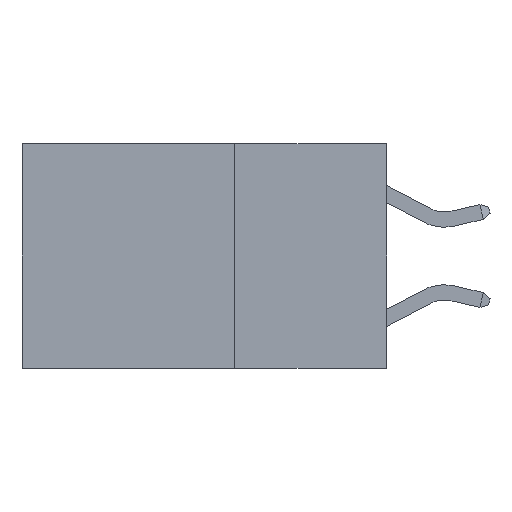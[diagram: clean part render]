
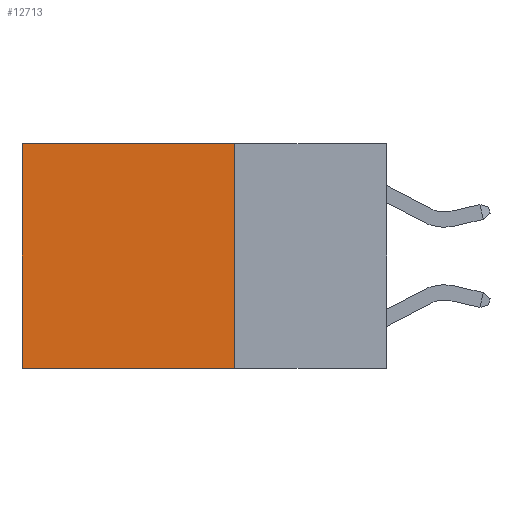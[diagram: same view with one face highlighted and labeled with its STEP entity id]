
A CAD part, left-side view. The second image highlights one B-rep face of the part: STEP entity #12713.
In plain terms, the highlighted planar face has unit normal (-1, 0, 0).
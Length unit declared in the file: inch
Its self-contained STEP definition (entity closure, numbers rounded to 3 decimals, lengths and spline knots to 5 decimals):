
#33 = EDGE_CURVE ( 'NONE', #10007, #8525, #7370, .T. ) ;
#2147 = VECTOR ( 'NONE', #4377, 39.37008 ) ;
#2740 = AXIS2_PLACEMENT_3D ( 'NONE', #23702, #5117, #19915 ) ;
#2826 = LINE ( 'NONE', #7041, #7732 ) ;
#2960 = DIRECTION ( 'NONE',  ( 0., 0., -1. ) ) ;
#3546 = CARTESIAN_POINT ( 'NONE',  ( 0.2625, 0.25, 0. ) ) ;
#3623 = EDGE_CURVE ( 'NONE', #10125, #24900, #12523, .T. ) ;
#3846 = CARTESIAN_POINT ( 'NONE',  ( 0.2625, 0.25, 0. ) ) ;
#4236 = ORIENTED_EDGE ( 'NONE', *, *, #3623, .F. ) ;
#4377 = DIRECTION ( 'NONE',  ( 0., 1., 0. ) ) ;
#5117 = DIRECTION ( 'NONE',  ( 1., 0., 0. ) ) ;
#5480 = DIRECTION ( 'NONE',  ( 0., 0., -1. ) ) ;
#7041 = CARTESIAN_POINT ( 'NONE',  ( 0.2625, 0.6, 0. ) ) ;
#7370 = LINE ( 'NONE', #3546, #26681 ) ;
#7568 = EDGE_CURVE ( 'NONE', #8525, #24900, #2826, .T. ) ;
#7732 = VECTOR ( 'NONE', #2960, 39.37008 ) ;
#8525 = VERTEX_POINT ( 'NONE', #21170 ) ;
#9175 = EDGE_LOOP ( 'NONE', ( #9224, #4236, #25086, #16341 ) ) ;
#9195 = PLANE ( 'NONE',  #2740 ) ;
#9224 = ORIENTED_EDGE ( 'NONE', *, *, #7568, .T. ) ;
#10007 = VERTEX_POINT ( 'NONE', #23346 ) ;
#10125 = VERTEX_POINT ( 'NONE', #13298 ) ;
#10482 = CARTESIAN_POINT ( 'NONE',  ( 0.2625, 0.25, -0.37 ) ) ;
#12523 = LINE ( 'NONE', #10482, #2147 ) ;
#12713 = ADVANCED_FACE ( 'NONE', ( #17735 ), #9195, .F. ) ;
#13298 = CARTESIAN_POINT ( 'NONE',  ( 0.2625, 0.25, -0.37 ) ) ;
#13317 = DIRECTION ( 'NONE',  ( 0., 1., 0. ) ) ;
#16341 = ORIENTED_EDGE ( 'NONE', *, *, #33, .T. ) ;
#16844 = EDGE_CURVE ( 'NONE', #10007, #10125, #22029, .T. ) ;
#17409 = CARTESIAN_POINT ( 'NONE',  ( 0.2625, 0.6, -0.37 ) ) ;
#17735 = FACE_OUTER_BOUND ( 'NONE', #9175, .T. ) ;
#19915 = DIRECTION ( 'NONE',  ( 0., 0., -1. ) ) ;
#21170 = CARTESIAN_POINT ( 'NONE',  ( 0.2625, 0.6, 0. ) ) ;
#22029 = LINE ( 'NONE', #3846, #25856 ) ;
#23346 = CARTESIAN_POINT ( 'NONE',  ( 0.2625, 0.25, 0. ) ) ;
#23702 = CARTESIAN_POINT ( 'NONE',  ( 0.2625, 0.25, 0. ) ) ;
#24900 = VERTEX_POINT ( 'NONE', #17409 ) ;
#25086 = ORIENTED_EDGE ( 'NONE', *, *, #16844, .F. ) ;
#25856 = VECTOR ( 'NONE', #5480, 39.37008 ) ;
#26681 = VECTOR ( 'NONE', #13317, 39.37008 ) ;
